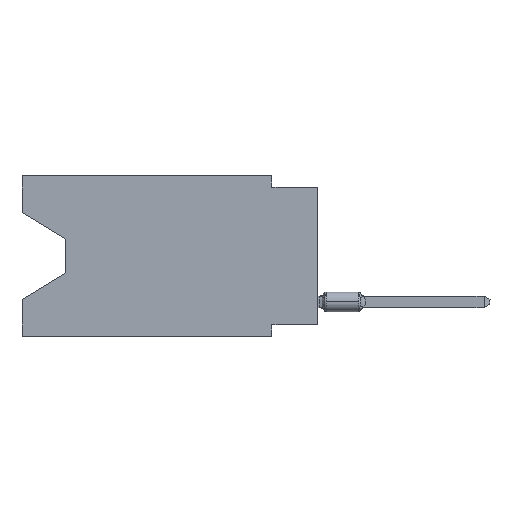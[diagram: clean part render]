
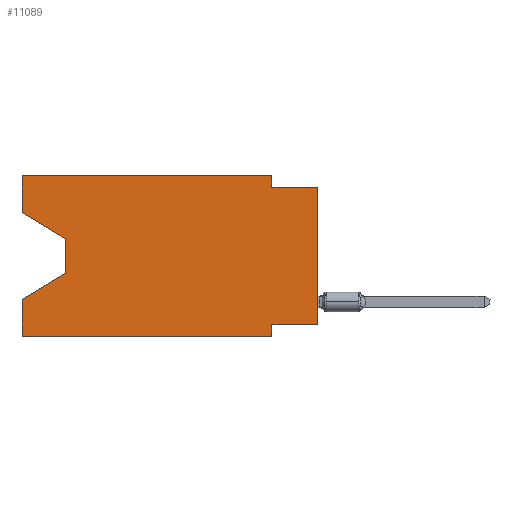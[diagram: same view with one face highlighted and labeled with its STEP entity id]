
A CAD part, left-side view. The second image highlights one B-rep face of the part: STEP entity #11089.
In plain terms, the highlighted planar face has unit normal (-1, 0, 0).
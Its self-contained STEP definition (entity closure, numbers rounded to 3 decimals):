
#478 = EDGE_CURVE ( 'NONE', #16040, #9366, #15879, .T. ) ;
#539 = CARTESIAN_POINT ( 'NONE',  ( 0., 2.54, -8.89 ) ) ;
#596 = VECTOR ( 'NONE', #4687, 1000. ) ;
#778 = CARTESIAN_POINT ( 'NONE',  ( 0., 13.97, -3.505 ) ) ;
#780 = LINE ( 'NONE', #8923, #4559 ) ;
#872 = VERTEX_POINT ( 'NONE', #13035 ) ;
#1018 = ORIENTED_EDGE ( 'NONE', *, *, #8354, .T. ) ;
#1055 = ORIENTED_EDGE ( 'NONE', *, *, #15278, .T. ) ;
#1292 = CARTESIAN_POINT ( 'NONE',  ( 0., 16.383, -8.89 ) ) ;
#1651 = DIRECTION ( 'NONE',  ( 0., -1., 0. ) ) ;
#1655 = VECTOR ( 'NONE', #1651, 1000. ) ;
#2010 = CARTESIAN_POINT ( 'NONE',  ( 0., 16.383, 0. ) ) ;
#2066 = CARTESIAN_POINT ( 'NONE',  ( 0., 13.97, -5.385 ) ) ;
#2284 = DIRECTION ( 'NONE',  ( 0., 1., 0. ) ) ;
#2562 = EDGE_CURVE ( 'NONE', #8599, #14516, #17074, .T. ) ;
#2603 = VERTEX_POINT ( 'NONE', #9535 ) ;
#2668 = VERTEX_POINT ( 'NONE', #10799 ) ;
#2858 = ORIENTED_EDGE ( 'NONE', *, *, #478, .F. ) ;
#2889 = CARTESIAN_POINT ( 'NONE',  ( 0., 13.97, -3.505 ) ) ;
#3028 = DIRECTION ( 'NONE',  ( 0., 0., 1. ) ) ;
#3149 = ORIENTED_EDGE ( 'NONE', *, *, #6019, .F. ) ;
#3309 = DIRECTION ( 'NONE',  ( 0., 0., 1. ) ) ;
#3561 = LINE ( 'NONE', #14663, #17795 ) ;
#3989 = CARTESIAN_POINT ( 'NONE',  ( 0., 0., -8.255 ) ) ;
#4389 = LINE ( 'NONE', #7178, #5535 ) ;
#4488 = EDGE_CURVE ( 'NONE', #2603, #7090, #10230, .T. ) ;
#4517 = CARTESIAN_POINT ( 'NONE',  ( 0., 2.54, -0.635 ) ) ;
#4518 = ORIENTED_EDGE ( 'NONE', *, *, #2562, .T. ) ;
#4559 = VECTOR ( 'NONE', #10452, 1000. ) ;
#4625 = LINE ( 'NONE', #17266, #13191 ) ;
#4687 = DIRECTION ( 'NONE',  ( 0., 0., -1. ) ) ;
#4696 = EDGE_CURVE ( 'NONE', #14516, #7090, #10839, .T. ) ;
#4885 = ORIENTED_EDGE ( 'NONE', *, *, #4696, .T. ) ;
#4891 = DIRECTION ( 'NONE',  ( 0., 0., -1. ) ) ;
#4984 = EDGE_CURVE ( 'NONE', #5575, #16037, #4625, .T. ) ;
#5374 = FACE_OUTER_BOUND ( 'NONE', #6650, .T. ) ;
#5499 = EDGE_CURVE ( 'NONE', #9366, #5575, #6277, .T. ) ;
#5535 = VECTOR ( 'NONE', #3028, 1000. ) ;
#5575 = VERTEX_POINT ( 'NONE', #15609 ) ;
#5641 = DIRECTION ( 'NONE',  ( 1., 0., 0. ) ) ;
#5878 = CARTESIAN_POINT ( 'NONE',  ( 0., 16.383, -2.038 ) ) ;
#5905 = EDGE_CURVE ( 'NONE', #16037, #872, #780, .T. ) ;
#6019 = EDGE_CURVE ( 'NONE', #2668, #17351, #17771, .T. ) ;
#6277 = LINE ( 'NONE', #8801, #7992 ) ;
#6650 = EDGE_LOOP ( 'NONE', ( #1018, #4518, #4885, #7806, #13139, #3149, #15051, #1055, #16253, #11904, #15326, #2858 ) ) ;
#6997 = PLANE ( 'NONE',  #13933 ) ;
#7090 = VERTEX_POINT ( 'NONE', #14464 ) ;
#7178 = CARTESIAN_POINT ( 'NONE',  ( 0., 0., 0. ) ) ;
#7766 = EDGE_CURVE ( 'NONE', #2603, #17351, #11058, .T. ) ;
#7806 = ORIENTED_EDGE ( 'NONE', *, *, #4488, .F. ) ;
#7992 = VECTOR ( 'NONE', #14143, 1000. ) ;
#8010 = VECTOR ( 'NONE', #9537, 1000. ) ;
#8016 = VERTEX_POINT ( 'NONE', #3989 ) ;
#8354 = EDGE_CURVE ( 'NONE', #16040, #8599, #14466, .T. ) ;
#8599 = VERTEX_POINT ( 'NONE', #2889 ) ;
#8801 = CARTESIAN_POINT ( 'NONE',  ( 0., 16.383, 0. ) ) ;
#8923 = CARTESIAN_POINT ( 'NONE',  ( 0., 0., -0.635 ) ) ;
#9113 = EDGE_CURVE ( 'NONE', #8016, #2668, #3561, .T. ) ;
#9288 = CARTESIAN_POINT ( 'NONE',  ( 0., 16.383, 0. ) ) ;
#9366 = VERTEX_POINT ( 'NONE', #9288 ) ;
#9535 = CARTESIAN_POINT ( 'NONE',  ( 0., 16.383, -8.89 ) ) ;
#9537 = DIRECTION ( 'NONE',  ( 0., 0., -1. ) ) ;
#10230 = LINE ( 'NONE', #2010, #16736 ) ;
#10316 = DIRECTION ( 'NONE',  ( 0., 0., 1. ) ) ;
#10452 = DIRECTION ( 'NONE',  ( 0., -1., 0. ) ) ;
#10799 = CARTESIAN_POINT ( 'NONE',  ( 0., 2.54, -8.255 ) ) ;
#10839 = LINE ( 'NONE', #14657, #11830 ) ;
#10858 = VECTOR ( 'NONE', #14556, 1000. ) ;
#11058 = LINE ( 'NONE', #1292, #1655 ) ;
#11089 = ADVANCED_FACE ( 'NONE', ( #5374 ), #6997, .F. ) ;
#11830 = VECTOR ( 'NONE', #16370, 1000. ) ;
#11904 = ORIENTED_EDGE ( 'NONE', *, *, #4984, .F. ) ;
#11999 = VECTOR ( 'NONE', #3309, 1000. ) ;
#12516 = CARTESIAN_POINT ( 'NONE',  ( 0., 16.383, 0. ) ) ;
#13035 = CARTESIAN_POINT ( 'NONE',  ( 0., 0., -0.635 ) ) ;
#13139 = ORIENTED_EDGE ( 'NONE', *, *, #7766, .T. ) ;
#13191 = VECTOR ( 'NONE', #4891, 1000. ) ;
#13933 = AXIS2_PLACEMENT_3D ( 'NONE', #12516, #5641, #16672 ) ;
#14143 = DIRECTION ( 'NONE',  ( 0., -1., 0. ) ) ;
#14287 = CARTESIAN_POINT ( 'NONE',  ( 0., 16.383, -2.038 ) ) ;
#14464 = CARTESIAN_POINT ( 'NONE',  ( 0., 16.383, -6.852 ) ) ;
#14466 = LINE ( 'NONE', #14287, #10858 ) ;
#14516 = VERTEX_POINT ( 'NONE', #2066 ) ;
#14556 = DIRECTION ( 'NONE',  ( 0., -0.855, -0.519 ) ) ;
#14657 = CARTESIAN_POINT ( 'NONE',  ( 0., 13.97, -5.385 ) ) ;
#14663 = CARTESIAN_POINT ( 'NONE',  ( 0., 0., -8.255 ) ) ;
#15051 = ORIENTED_EDGE ( 'NONE', *, *, #9113, .F. ) ;
#15060 = CARTESIAN_POINT ( 'NONE',  ( 0., 2.54, -8.89 ) ) ;
#15278 = EDGE_CURVE ( 'NONE', #8016, #872, #4389, .T. ) ;
#15326 = ORIENTED_EDGE ( 'NONE', *, *, #5499, .F. ) ;
#15609 = CARTESIAN_POINT ( 'NONE',  ( 0., 2.54, 0. ) ) ;
#15613 = CARTESIAN_POINT ( 'NONE',  ( 0., 16.383, 0. ) ) ;
#15879 = LINE ( 'NONE', #15613, #11999 ) ;
#16037 = VERTEX_POINT ( 'NONE', #4517 ) ;
#16040 = VERTEX_POINT ( 'NONE', #5878 ) ;
#16253 = ORIENTED_EDGE ( 'NONE', *, *, #5905, .F. ) ;
#16370 = DIRECTION ( 'NONE',  ( 0., 0.855, -0.519 ) ) ;
#16672 = DIRECTION ( 'NONE',  ( 0., 0., -1. ) ) ;
#16736 = VECTOR ( 'NONE', #10316, 1000. ) ;
#17074 = LINE ( 'NONE', #778, #596 ) ;
#17266 = CARTESIAN_POINT ( 'NONE',  ( 0., 2.54, 0. ) ) ;
#17351 = VERTEX_POINT ( 'NONE', #539 ) ;
#17771 = LINE ( 'NONE', #15060, #8010 ) ;
#17795 = VECTOR ( 'NONE', #2284, 1000. ) ;
